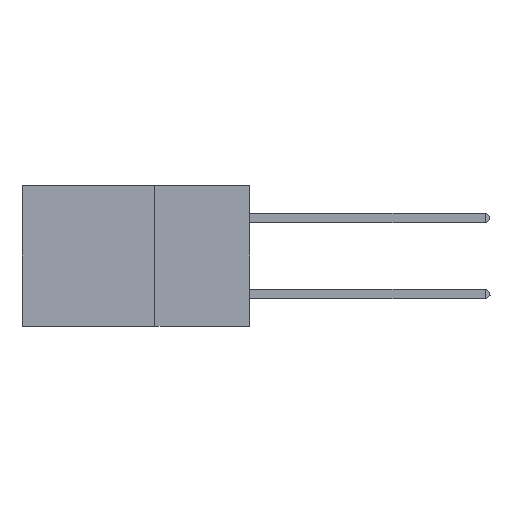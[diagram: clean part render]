
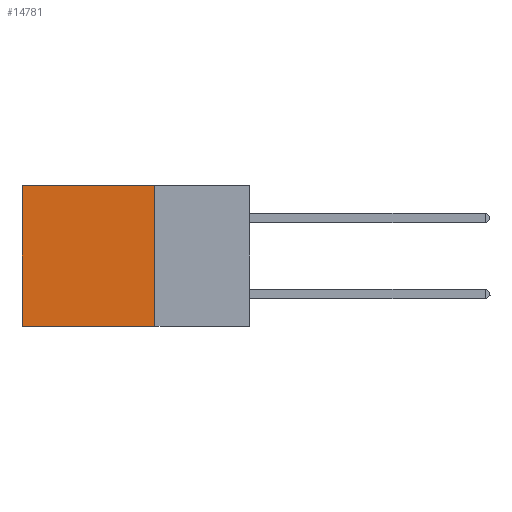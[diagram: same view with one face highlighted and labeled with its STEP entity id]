
A CAD part, left-side view. The second image highlights one B-rep face of the part: STEP entity #14781.
In plain terms, the highlighted planar face has unit normal (-1, 0, 0).
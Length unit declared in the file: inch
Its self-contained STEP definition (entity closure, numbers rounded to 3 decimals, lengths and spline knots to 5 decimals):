
#680 = LINE ( 'NONE', #21334, #27858 ) ;
#1372 = VECTOR ( 'NONE', #20014, 39.37008 ) ;
#2357 = ORIENTED_EDGE ( 'NONE', *, *, #10484, .T. ) ;
#3005 = LINE ( 'NONE', #27284, #1372 ) ;
#3382 = DIRECTION ( 'NONE',  ( 0., 0., -1. ) ) ;
#3984 = PLANE ( 'NONE',  #33236 ) ;
#4211 = DIRECTION ( 'NONE',  ( 1., 0., 0. ) ) ;
#5358 = VERTEX_POINT ( 'NONE', #15660 ) ;
#9202 = VERTEX_POINT ( 'NONE', #28585 ) ;
#9590 = VECTOR ( 'NONE', #22363, 39.37008 ) ;
#10294 = EDGE_LOOP ( 'NONE', ( #14443, #23893, #15661, #2357 ) ) ;
#10484 = EDGE_CURVE ( 'NONE', #5358, #9202, #680, .T. ) ;
#14047 = VERTEX_POINT ( 'NONE', #16030 ) ;
#14443 = ORIENTED_EDGE ( 'NONE', *, *, #30619, .T. ) ;
#14781 = ADVANCED_FACE ( 'NONE', ( #33302 ), #3984, .F. ) ;
#15660 = CARTESIAN_POINT ( 'NONE',  ( 0.2875, 0.25, 0. ) ) ;
#15661 = ORIENTED_EDGE ( 'NONE', *, *, #21305, .F. ) ;
#16030 = CARTESIAN_POINT ( 'NONE',  ( 0.2875, 0.6, -0.37 ) ) ;
#16313 = CARTESIAN_POINT ( 'NONE',  ( 0.2875, 0.6, 0. ) ) ;
#16785 = CARTESIAN_POINT ( 'NONE',  ( 0.2875, 0.25, -0.37 ) ) ;
#16893 = CARTESIAN_POINT ( 'NONE',  ( 0.2875, 0.25, 0. ) ) ;
#19403 = DIRECTION ( 'NONE',  ( 0., 0., -1. ) ) ;
#20014 = DIRECTION ( 'NONE',  ( 0., 0., -1. ) ) ;
#20185 = EDGE_CURVE ( 'NONE', #26841, #14047, #25032, .T. ) ;
#21305 = EDGE_CURVE ( 'NONE', #5358, #26841, #3005, .T. ) ;
#21334 = CARTESIAN_POINT ( 'NONE',  ( 0.2875, 0.25, 0. ) ) ;
#22363 = DIRECTION ( 'NONE',  ( 0., 1., 0. ) ) ;
#23893 = ORIENTED_EDGE ( 'NONE', *, *, #20185, .F. ) ;
#25032 = LINE ( 'NONE', #27459, #9590 ) ;
#26841 = VERTEX_POINT ( 'NONE', #16785 ) ;
#27284 = CARTESIAN_POINT ( 'NONE',  ( 0.2875, 0.25, 0. ) ) ;
#27459 = CARTESIAN_POINT ( 'NONE',  ( 0.2875, 0.25, -0.37 ) ) ;
#27858 = VECTOR ( 'NONE', #31762, 39.37008 ) ;
#28261 = LINE ( 'NONE', #16313, #31099 ) ;
#28585 = CARTESIAN_POINT ( 'NONE',  ( 0.2875, 0.6, 0. ) ) ;
#30619 = EDGE_CURVE ( 'NONE', #9202, #14047, #28261, .T. ) ;
#31099 = VECTOR ( 'NONE', #3382, 39.37008 ) ;
#31762 = DIRECTION ( 'NONE',  ( 0., 1., 0. ) ) ;
#33236 = AXIS2_PLACEMENT_3D ( 'NONE', #16893, #4211, #19403 ) ;
#33302 = FACE_OUTER_BOUND ( 'NONE', #10294, .T. ) ;
